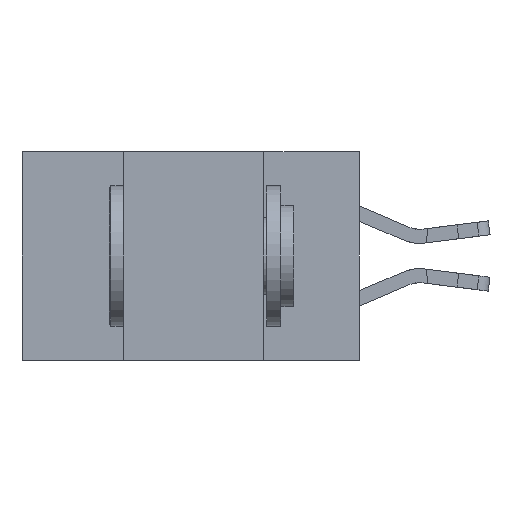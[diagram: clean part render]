
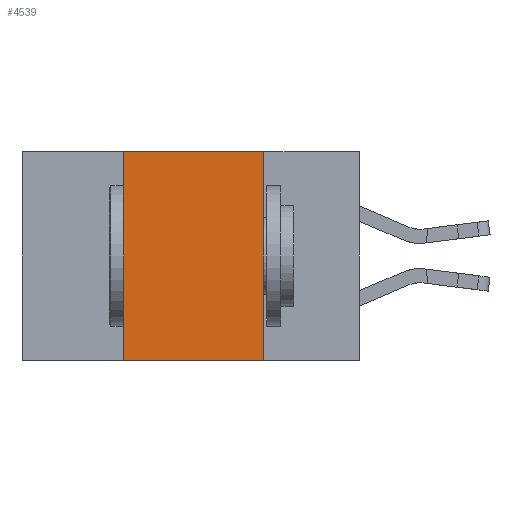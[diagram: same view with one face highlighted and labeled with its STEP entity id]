
A CAD part, left-side view. The second image highlights one B-rep face of the part: STEP entity #4539.
In plain terms, the highlighted planar face has unit normal (-1, 0, 0).
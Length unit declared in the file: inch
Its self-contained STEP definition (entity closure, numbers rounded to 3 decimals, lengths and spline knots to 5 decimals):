
#201 = VERTEX_POINT ( 'NONE', #16675 ) ;
#258 = EDGE_CURVE ( 'NONE', #6657, #2411, #14298, .T. ) ;
#1182 = CARTESIAN_POINT ( 'NONE',  ( 0., 0.17, -0.37 ) ) ;
#1826 = DIRECTION ( 'NONE',  ( 0., 0., -1. ) ) ;
#1923 = LINE ( 'NONE', #4164, #16474 ) ;
#2371 = VECTOR ( 'NONE', #16865, 39.37008 ) ;
#2411 = VERTEX_POINT ( 'NONE', #1182 ) ;
#2437 = EDGE_LOOP ( 'NONE', ( #8550, #5935, #6009, #16427 ) ) ;
#2614 = CARTESIAN_POINT ( 'NONE',  ( 0., 0.6, -0.37 ) ) ;
#3782 = CARTESIAN_POINT ( 'NONE',  ( 0., 0.6, 0. ) ) ;
#4164 = CARTESIAN_POINT ( 'NONE',  ( 0., 0.42, 0. ) ) ;
#4539 = ADVANCED_FACE ( 'NONE', ( #10330 ), #19277, .F. ) ;
#5222 = DIRECTION ( 'NONE',  ( 0., 0., -1. ) ) ;
#5935 = ORIENTED_EDGE ( 'NONE', *, *, #7275, .F. ) ;
#6009 = ORIENTED_EDGE ( 'NONE', *, *, #19123, .F. ) ;
#6395 = VERTEX_POINT ( 'NONE', #6783 ) ;
#6657 = VERTEX_POINT ( 'NONE', #16344 ) ;
#6783 = CARTESIAN_POINT ( 'NONE',  ( 0., 0.42, -0.37 ) ) ;
#7123 = VECTOR ( 'NONE', #1826, 39.37008 ) ;
#7275 = EDGE_CURVE ( 'NONE', #201, #6657, #18435, .T. ) ;
#8136 = CARTESIAN_POINT ( 'NONE',  ( 0., 0.17, 0. ) ) ;
#8550 = ORIENTED_EDGE ( 'NONE', *, *, #258, .F. ) ;
#9037 = LINE ( 'NONE', #2614, #16408 ) ;
#10330 = FACE_OUTER_BOUND ( 'NONE', #2437, .T. ) ;
#14298 = LINE ( 'NONE', #8136, #7123 ) ;
#15195 = DIRECTION ( 'NONE',  ( 0., 0., 1. ) ) ;
#15484 = CARTESIAN_POINT ( 'NONE',  ( 0., 0.6, 0. ) ) ;
#16344 = CARTESIAN_POINT ( 'NONE',  ( 0., 0.17, 0. ) ) ;
#16408 = VECTOR ( 'NONE', #19837, 39.37008 ) ;
#16427 = ORIENTED_EDGE ( 'NONE', *, *, #20361, .T. ) ;
#16474 = VECTOR ( 'NONE', #15195, 39.37008 ) ;
#16675 = CARTESIAN_POINT ( 'NONE',  ( 0., 0.42, 0. ) ) ;
#16865 = DIRECTION ( 'NONE',  ( 0., -1., 0. ) ) ;
#17359 = AXIS2_PLACEMENT_3D ( 'NONE', #3782, #17989, #5222 ) ;
#17989 = DIRECTION ( 'NONE',  ( 1., 0., 0. ) ) ;
#18435 = LINE ( 'NONE', #15484, #2371 ) ;
#19123 = EDGE_CURVE ( 'NONE', #6395, #201, #1923, .T. ) ;
#19277 = PLANE ( 'NONE',  #17359 ) ;
#19837 = DIRECTION ( 'NONE',  ( 0., -1., 0. ) ) ;
#20361 = EDGE_CURVE ( 'NONE', #6395, #2411, #9037, .T. ) ;
